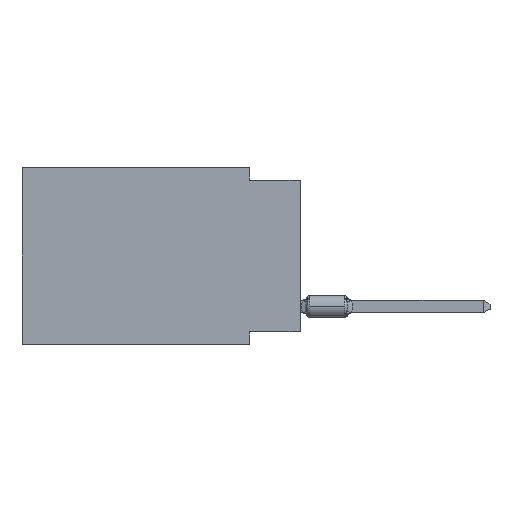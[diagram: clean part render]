
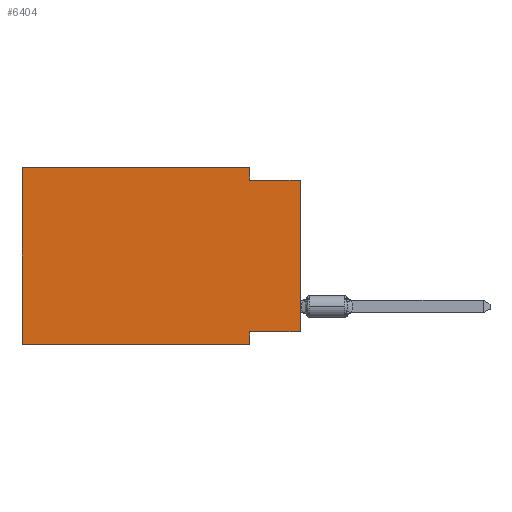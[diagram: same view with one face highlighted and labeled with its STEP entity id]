
A CAD part, left-side view. The second image highlights one B-rep face of the part: STEP entity #6404.
In plain terms, the highlighted planar face has unit normal (-1, 0, 0).
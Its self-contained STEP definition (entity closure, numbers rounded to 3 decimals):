
#192 = VECTOR ( 'NONE', #17897, 1000. ) ;
#578 = VERTEX_POINT ( 'NONE', #22486 ) ;
#1166 = VERTEX_POINT ( 'NONE', #8608 ) ;
#1510 = VERTEX_POINT ( 'NONE', #20579 ) ;
#1636 = EDGE_CURVE ( 'NONE', #578, #1510, #11491, .T. ) ;
#1704 = ORIENTED_EDGE ( 'NONE', *, *, #9575, .T. ) ;
#2444 = CARTESIAN_POINT ( 'NONE',  ( 0., 13.97, 0. ) ) ;
#2804 = EDGE_CURVE ( 'NONE', #16621, #1166, #14661, .T. ) ;
#4319 = VERTEX_POINT ( 'NONE', #12126 ) ;
#4442 = ORIENTED_EDGE ( 'NONE', *, *, #11764, .F. ) ;
#4464 = EDGE_CURVE ( 'NONE', #18288, #578, #11829, .T. ) ;
#5125 = DIRECTION ( 'NONE',  ( 0., 0., -1. ) ) ;
#6139 = CARTESIAN_POINT ( 'NONE',  ( 0., 2.54, 0. ) ) ;
#6404 = ADVANCED_FACE ( 'NONE', ( #6577 ), #15905, .F. ) ;
#6495 = ORIENTED_EDGE ( 'NONE', *, *, #4464, .F. ) ;
#6577 = FACE_OUTER_BOUND ( 'NONE', #7330, .T. ) ;
#7061 = ORIENTED_EDGE ( 'NONE', *, *, #1636, .F. ) ;
#7330 = EDGE_LOOP ( 'NONE', ( #1704, #4442, #15953, #7061, #6495, #16859, #8488, #8474 ) ) ;
#7445 = VERTEX_POINT ( 'NONE', #15555 ) ;
#8271 = DIRECTION ( 'NONE',  ( 1., 0., 0. ) ) ;
#8474 = ORIENTED_EDGE ( 'NONE', *, *, #19135, .F. ) ;
#8488 = ORIENTED_EDGE ( 'NONE', *, *, #2804, .F. ) ;
#8578 = DIRECTION ( 'NONE',  ( 0., -1., 0. ) ) ;
#8608 = CARTESIAN_POINT ( 'NONE',  ( 0., 2.54, -8.89 ) ) ;
#9084 = DIRECTION ( 'NONE',  ( 0., 0., -1. ) ) ;
#9575 = EDGE_CURVE ( 'NONE', #4319, #9760, #11778, .T. ) ;
#9760 = VERTEX_POINT ( 'NONE', #22296 ) ;
#10262 = CARTESIAN_POINT ( 'NONE',  ( 0., 0., -8.255 ) ) ;
#11116 = VECTOR ( 'NONE', #17058, 1000. ) ;
#11491 = LINE ( 'NONE', #2444, #16115 ) ;
#11764 = EDGE_CURVE ( 'NONE', #7445, #9760, #16106, .T. ) ;
#11778 = LINE ( 'NONE', #22687, #17091 ) ;
#11829 = LINE ( 'NONE', #22740, #11116 ) ;
#11847 = DIRECTION ( 'NONE',  ( 0., -1., 0. ) ) ;
#12126 = CARTESIAN_POINT ( 'NONE',  ( 0., 0., -8.255 ) ) ;
#13623 = DIRECTION ( 'NONE',  ( 0., 0., -1. ) ) ;
#13671 = EDGE_CURVE ( 'NONE', #18288, #1166, #17761, .T. ) ;
#14008 = DIRECTION ( 'NONE',  ( 0., -1., 0. ) ) ;
#14661 = LINE ( 'NONE', #22160, #23040 ) ;
#15546 = CARTESIAN_POINT ( 'NONE',  ( 0., 2.54, -8.255 ) ) ;
#15555 = CARTESIAN_POINT ( 'NONE',  ( 0., 2.54, -0.635 ) ) ;
#15905 = PLANE ( 'NONE',  #16273 ) ;
#15953 = ORIENTED_EDGE ( 'NONE', *, *, #17215, .F. ) ;
#16106 = LINE ( 'NONE', #17785, #16179 ) ;
#16115 = VECTOR ( 'NONE', #11847, 1000. ) ;
#16179 = VECTOR ( 'NONE', #8578, 1000. ) ;
#16273 = AXIS2_PLACEMENT_3D ( 'NONE', #19640, #8271, #5125 ) ;
#16621 = VERTEX_POINT ( 'NONE', #15546 ) ;
#16759 = VECTOR ( 'NONE', #13623, 1000. ) ;
#16859 = ORIENTED_EDGE ( 'NONE', *, *, #13671, .T. ) ;
#17009 = DIRECTION ( 'NONE',  ( 0., 0., 1. ) ) ;
#17058 = DIRECTION ( 'NONE',  ( 0., 0., 1. ) ) ;
#17091 = VECTOR ( 'NONE', #17009, 1000. ) ;
#17215 = EDGE_CURVE ( 'NONE', #1510, #7445, #19637, .T. ) ;
#17761 = LINE ( 'NONE', #19921, #19695 ) ;
#17785 = CARTESIAN_POINT ( 'NONE',  ( 0., 0., -0.635 ) ) ;
#17897 = DIRECTION ( 'NONE',  ( 0., 1., 0. ) ) ;
#18288 = VERTEX_POINT ( 'NONE', #20534 ) ;
#19135 = EDGE_CURVE ( 'NONE', #4319, #16621, #19585, .T. ) ;
#19585 = LINE ( 'NONE', #10262, #192 ) ;
#19637 = LINE ( 'NONE', #6139, #16759 ) ;
#19640 = CARTESIAN_POINT ( 'NONE',  ( 0., 13.97, 0. ) ) ;
#19695 = VECTOR ( 'NONE', #14008, 1000. ) ;
#19921 = CARTESIAN_POINT ( 'NONE',  ( 0., 13.97, -8.89 ) ) ;
#20534 = CARTESIAN_POINT ( 'NONE',  ( 0., 13.97, -8.89 ) ) ;
#20579 = CARTESIAN_POINT ( 'NONE',  ( 0., 2.54, 0. ) ) ;
#22160 = CARTESIAN_POINT ( 'NONE',  ( 0., 2.54, -8.89 ) ) ;
#22296 = CARTESIAN_POINT ( 'NONE',  ( 0., 0., -0.635 ) ) ;
#22486 = CARTESIAN_POINT ( 'NONE',  ( 0., 13.97, 0. ) ) ;
#22687 = CARTESIAN_POINT ( 'NONE',  ( 0., 0., 0. ) ) ;
#22740 = CARTESIAN_POINT ( 'NONE',  ( 0., 13.97, 0. ) ) ;
#23040 = VECTOR ( 'NONE', #9084, 1000. ) ;
